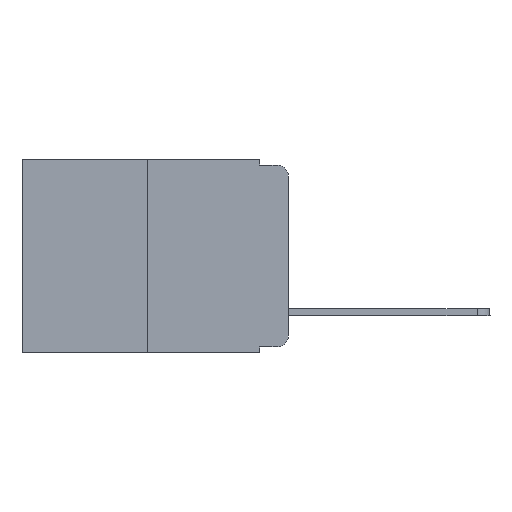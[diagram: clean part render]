
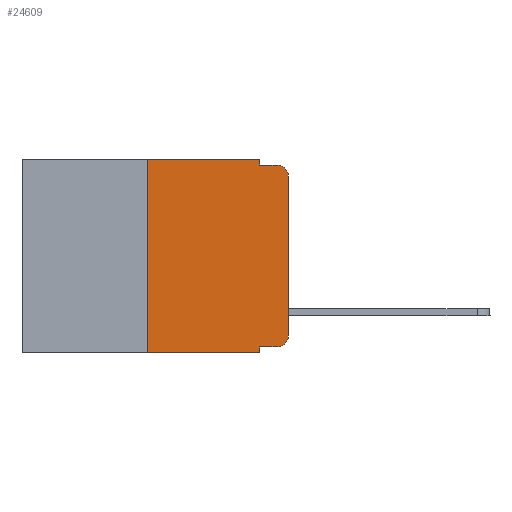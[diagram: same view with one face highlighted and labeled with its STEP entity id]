
A CAD part, left-side view. The second image highlights one B-rep face of the part: STEP entity #24609.
In plain terms, the highlighted planar face has unit normal (-1, 0, 0).
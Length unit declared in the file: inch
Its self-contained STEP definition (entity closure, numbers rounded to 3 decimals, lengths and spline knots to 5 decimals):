
#187 = DIRECTION ( 'NONE',  ( 0., -1., 0. ) ) ;
#396 = ORIENTED_EDGE ( 'NONE', *, *, #22382, .T. ) ;
#719 = EDGE_CURVE ( 'NONE', #16681, #3171, #5388, .T. ) ;
#924 = VECTOR ( 'NONE', #4360, 39.37008 ) ;
#1473 = LINE ( 'NONE', #22978, #17816 ) ;
#1957 = EDGE_CURVE ( 'NONE', #20511, #11363, #1473, .T. ) ;
#2342 = ORIENTED_EDGE ( 'NONE', *, *, #21175, .F. ) ;
#2356 = CARTESIAN_POINT ( 'NONE',  ( 0., 0.051, 0. ) ) ;
#3007 = VECTOR ( 'NONE', #7315, 39.37008 ) ;
#3104 = CARTESIAN_POINT ( 'NONE',  ( 0., 0.051, -0.01 ) ) ;
#3171 = VERTEX_POINT ( 'NONE', #8569 ) ;
#3315 = AXIS2_PLACEMENT_3D ( 'NONE', #19435, #9974, #23259 ) ;
#4160 = ORIENTED_EDGE ( 'NONE', *, *, #18788, .F. ) ;
#4328 = CARTESIAN_POINT ( 'NONE',  ( 0., 0.473, 0. ) ) ;
#4360 = DIRECTION ( 'NONE',  ( 0., 0., -1. ) ) ;
#4549 = LINE ( 'NONE', #18833, #5726 ) ;
#5053 = CIRCLE ( 'NONE', #12186, 0.02 ) ;
#5227 = DIRECTION ( 'NONE',  ( 0., -1., 0. ) ) ;
#5388 = LINE ( 'NONE', #21638, #24152 ) ;
#5726 = VECTOR ( 'NONE', #18672, 39.37008 ) ;
#6696 = VERTEX_POINT ( 'NONE', #2356 ) ;
#6737 = DIRECTION ( 'NONE',  ( 0., 0., 1. ) ) ;
#6739 = EDGE_CURVE ( 'NONE', #8710, #10431, #17647, .T. ) ;
#6830 = ORIENTED_EDGE ( 'NONE', *, *, #719, .T. ) ;
#6975 = CARTESIAN_POINT ( 'NONE',  ( 0., 0.051, -0.333 ) ) ;
#7315 = DIRECTION ( 'NONE',  ( 0., -1., 0. ) ) ;
#7587 = EDGE_LOOP ( 'NONE', ( #6830, #16801, #11879, #12275, #4160, #19973, #16405, #2342, #9957, #396 ) ) ;
#8205 = VERTEX_POINT ( 'NONE', #19073 ) ;
#8569 = CARTESIAN_POINT ( 'NONE',  ( 0., 0., -0.03 ) ) ;
#8710 = VERTEX_POINT ( 'NONE', #3104 ) ;
#8746 = CARTESIAN_POINT ( 'NONE',  ( 0., 0.25, 0. ) ) ;
#8761 = CARTESIAN_POINT ( 'NONE',  ( 0., 0.02, -0.313 ) ) ;
#8921 = CARTESIAN_POINT ( 'NONE',  ( 0., 0.051, -0.01 ) ) ;
#9680 = CARTESIAN_POINT ( 'NONE',  ( 0., 0.473, 0. ) ) ;
#9957 = ORIENTED_EDGE ( 'NONE', *, *, #22459, .T. ) ;
#9974 = DIRECTION ( 'NONE',  ( -1., 0., 0. ) ) ;
#10431 = VERTEX_POINT ( 'NONE', #23588 ) ;
#10968 = DIRECTION ( 'NONE',  ( 0., 0., 1. ) ) ;
#11363 = VERTEX_POINT ( 'NONE', #14948 ) ;
#11483 = CARTESIAN_POINT ( 'NONE',  ( 0., 0.25, -0.343 ) ) ;
#11879 = ORIENTED_EDGE ( 'NONE', *, *, #6739, .F. ) ;
#12186 = AXIS2_PLACEMENT_3D ( 'NONE', #8761, #23950, #12565 ) ;
#12275 = ORIENTED_EDGE ( 'NONE', *, *, #14224, .F. ) ;
#12565 = DIRECTION ( 'NONE',  ( 0., 0., -1. ) ) ;
#12910 = CARTESIAN_POINT ( 'NONE',  ( 0., 0.02, -0.333 ) ) ;
#13059 = CIRCLE ( 'NONE', #3315, 0.02 ) ;
#13883 = LINE ( 'NONE', #9680, #23402 ) ;
#14113 = EDGE_CURVE ( 'NONE', #20511, #14522, #14293, .T. ) ;
#14224 = EDGE_CURVE ( 'NONE', #6696, #8710, #23799, .T. ) ;
#14293 = LINE ( 'NONE', #8746, #15736 ) ;
#14522 = VERTEX_POINT ( 'NONE', #24006 ) ;
#14948 = CARTESIAN_POINT ( 'NONE',  ( 0., 0.051, -0.343 ) ) ;
#15118 = EDGE_CURVE ( 'NONE', #3171, #10431, #13059, .T. ) ;
#15400 = DIRECTION ( 'NONE',  ( 0., -1., 0. ) ) ;
#15601 = DIRECTION ( 'NONE',  ( 1., 0., 0. ) ) ;
#15688 = CARTESIAN_POINT ( 'NONE',  ( 0., 0.051, 0. ) ) ;
#15736 = VECTOR ( 'NONE', #10968, 39.37008 ) ;
#16405 = ORIENTED_EDGE ( 'NONE', *, *, #1957, .T. ) ;
#16681 = VERTEX_POINT ( 'NONE', #17499 ) ;
#16801 = ORIENTED_EDGE ( 'NONE', *, *, #15118, .T. ) ;
#17183 = FACE_OUTER_BOUND ( 'NONE', #7587, .T. ) ;
#17499 = CARTESIAN_POINT ( 'NONE',  ( 0., 0., -0.313 ) ) ;
#17647 = LINE ( 'NONE', #8921, #19457 ) ;
#17765 = DIRECTION ( 'NONE',  ( 0., 0., -1. ) ) ;
#17816 = VECTOR ( 'NONE', #15400, 39.37008 ) ;
#18571 = AXIS2_PLACEMENT_3D ( 'NONE', #4328, #15601, #17765 ) ;
#18672 = DIRECTION ( 'NONE',  ( 0., 0., -1. ) ) ;
#18788 = EDGE_CURVE ( 'NONE', #14522, #6696, #13883, .T. ) ;
#18833 = CARTESIAN_POINT ( 'NONE',  ( 0., 0.051, 0. ) ) ;
#19073 = CARTESIAN_POINT ( 'NONE',  ( 0., 0.051, -0.333 ) ) ;
#19435 = CARTESIAN_POINT ( 'NONE',  ( 0., 0.02, -0.03 ) ) ;
#19457 = VECTOR ( 'NONE', #5227, 39.37008 ) ;
#19528 = PLANE ( 'NONE',  #18571 ) ;
#19953 = LINE ( 'NONE', #6975, #3007 ) ;
#19973 = ORIENTED_EDGE ( 'NONE', *, *, #14113, .F. ) ;
#20511 = VERTEX_POINT ( 'NONE', #11483 ) ;
#21175 = EDGE_CURVE ( 'NONE', #8205, #11363, #4549, .T. ) ;
#21638 = CARTESIAN_POINT ( 'NONE',  ( 0., 0., 0. ) ) ;
#22382 = EDGE_CURVE ( 'NONE', #24234, #16681, #5053, .T. ) ;
#22459 = EDGE_CURVE ( 'NONE', #8205, #24234, #19953, .T. ) ;
#22978 = CARTESIAN_POINT ( 'NONE',  ( 0., 0.473, -0.343 ) ) ;
#23259 = DIRECTION ( 'NONE',  ( 0., 0., -1. ) ) ;
#23402 = VECTOR ( 'NONE', #187, 39.37008 ) ;
#23588 = CARTESIAN_POINT ( 'NONE',  ( 0., 0.02, -0.01 ) ) ;
#23799 = LINE ( 'NONE', #15688, #924 ) ;
#23950 = DIRECTION ( 'NONE',  ( -1., 0., 0. ) ) ;
#24006 = CARTESIAN_POINT ( 'NONE',  ( 0., 0.25, 0. ) ) ;
#24152 = VECTOR ( 'NONE', #6737, 39.37008 ) ;
#24234 = VERTEX_POINT ( 'NONE', #12910 ) ;
#24609 = ADVANCED_FACE ( 'NONE', ( #17183 ), #19528, .F. ) ;
